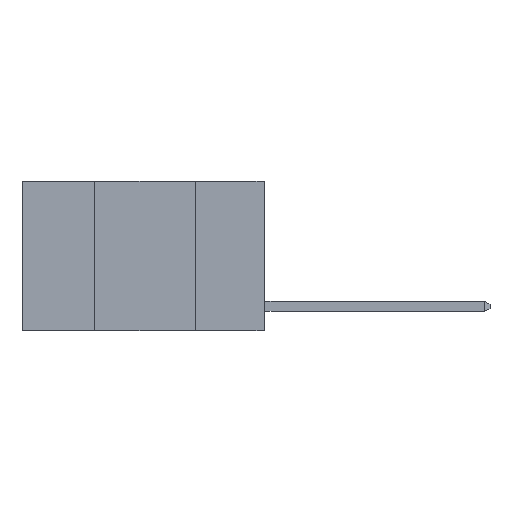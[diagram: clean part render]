
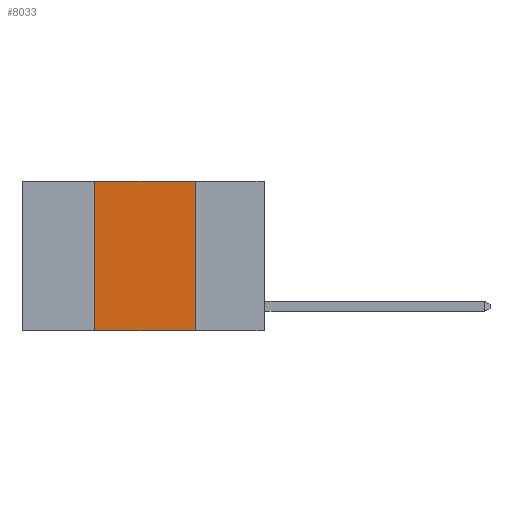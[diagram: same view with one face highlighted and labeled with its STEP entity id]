
A CAD part, left-side view. The second image highlights one B-rep face of the part: STEP entity #8033.
In plain terms, the highlighted planar face has unit normal (-1, 0, 0).
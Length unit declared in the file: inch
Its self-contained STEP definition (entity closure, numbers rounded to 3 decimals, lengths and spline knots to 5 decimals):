
#594 = DIRECTION ( 'NONE',  ( 0., 0., -1. ) ) ;
#714 = CARTESIAN_POINT ( 'NONE',  ( 0., 0.6, -0.37 ) ) ;
#1102 = DIRECTION ( 'NONE',  ( 0., 0., 1. ) ) ;
#1205 = EDGE_LOOP ( 'NONE', ( #6988, #2583, #4939, #7277 ) ) ;
#1279 = EDGE_CURVE ( 'NONE', #8958, #4562, #4615, .T. ) ;
#1389 = VECTOR ( 'NONE', #9559, 39.37008 ) ;
#1461 = EDGE_CURVE ( 'NONE', #9949, #8958, #8699, .T. ) ;
#2230 = VECTOR ( 'NONE', #1102, 39.37008 ) ;
#2297 = CARTESIAN_POINT ( 'NONE',  ( 0., 0.17, -0.37 ) ) ;
#2326 = CARTESIAN_POINT ( 'NONE',  ( 0., 0.42, 0. ) ) ;
#2583 = ORIENTED_EDGE ( 'NONE', *, *, #1279, .F. ) ;
#4156 = PLANE ( 'NONE',  #8035 ) ;
#4340 = CARTESIAN_POINT ( 'NONE',  ( 0., 0.17, 0. ) ) ;
#4562 = VERTEX_POINT ( 'NONE', #10335 ) ;
#4615 = LINE ( 'NONE', #8083, #9010 ) ;
#4657 = CARTESIAN_POINT ( 'NONE',  ( 0., 0.42, 0. ) ) ;
#4939 = ORIENTED_EDGE ( 'NONE', *, *, #1461, .F. ) ;
#5103 = VERTEX_POINT ( 'NONE', #2297 ) ;
#5687 = LINE ( 'NONE', #714, #10081 ) ;
#5897 = DIRECTION ( 'NONE',  ( 1., 0., 0. ) ) ;
#5904 = DIRECTION ( 'NONE',  ( 0., -1., 0. ) ) ;
#6889 = EDGE_CURVE ( 'NONE', #4562, #5103, #10495, .T. ) ;
#6988 = ORIENTED_EDGE ( 'NONE', *, *, #6889, .F. ) ;
#7246 = CARTESIAN_POINT ( 'NONE',  ( 0., 0.42, -0.37 ) ) ;
#7277 = ORIENTED_EDGE ( 'NONE', *, *, #7567, .T. ) ;
#7567 = EDGE_CURVE ( 'NONE', #9949, #5103, #5687, .T. ) ;
#7746 = FACE_OUTER_BOUND ( 'NONE', #1205, .T. ) ;
#7813 = DIRECTION ( 'NONE',  ( 0., -1., 0. ) ) ;
#8033 = ADVANCED_FACE ( 'NONE', ( #7746 ), #4156, .F. ) ;
#8035 = AXIS2_PLACEMENT_3D ( 'NONE', #10256, #5897, #594 ) ;
#8083 = CARTESIAN_POINT ( 'NONE',  ( 0., 0.6, 0. ) ) ;
#8699 = LINE ( 'NONE', #4657, #2230 ) ;
#8958 = VERTEX_POINT ( 'NONE', #2326 ) ;
#9010 = VECTOR ( 'NONE', #5904, 39.37008 ) ;
#9559 = DIRECTION ( 'NONE',  ( 0., 0., -1. ) ) ;
#9949 = VERTEX_POINT ( 'NONE', #7246 ) ;
#10081 = VECTOR ( 'NONE', #7813, 39.37008 ) ;
#10256 = CARTESIAN_POINT ( 'NONE',  ( 0., 0.6, 0. ) ) ;
#10335 = CARTESIAN_POINT ( 'NONE',  ( 0., 0.17, 0. ) ) ;
#10495 = LINE ( 'NONE', #4340, #1389 ) ;
